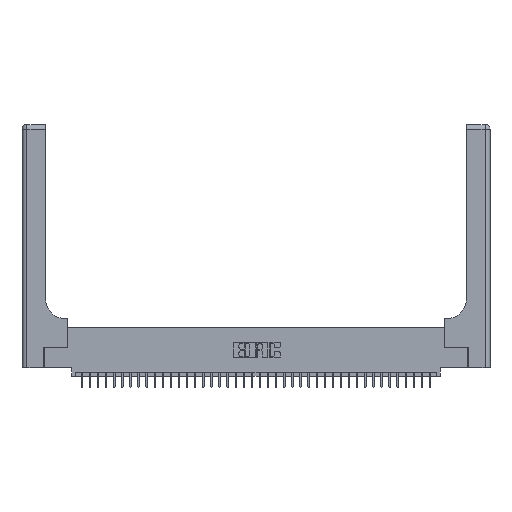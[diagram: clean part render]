
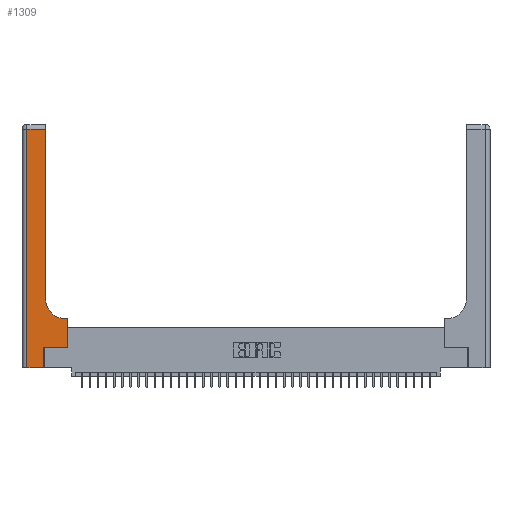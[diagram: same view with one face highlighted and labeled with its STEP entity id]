
A CAD part, top view. The second image highlights one B-rep face of the part: STEP entity #1309.
In plain terms, the highlighted planar face has unit normal (0, 0, 1).
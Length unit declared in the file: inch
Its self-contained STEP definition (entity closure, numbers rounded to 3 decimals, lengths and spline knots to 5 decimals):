
#410 = AXIS2_PLACEMENT_3D ( 'NONE', #12592, #3534, #15387 ) ;
#766 = DIRECTION ( 'NONE',  ( 0., 1., 0. ) ) ;
#1309 = ADVANCED_FACE ( 'NONE', ( #9378 ), #18802, .F. ) ;
#1773 = CARTESIAN_POINT ( 'NONE',  ( 0.06, 2.94, 0.37 ) ) ;
#2101 = LINE ( 'NONE', #14575, #7569 ) ;
#2392 = ORIENTED_EDGE ( 'NONE', *, *, #37537, .T. ) ;
#2927 = DIRECTION ( 'NONE',  ( 1., 0., 0. ) ) ;
#3534 = DIRECTION ( 'NONE',  ( 0., 0., -1. ) ) ;
#4312 = DIRECTION ( 'NONE',  ( 0., 1., 0. ) ) ;
#6578 = VECTOR ( 'NONE', #30595, 39.37008 ) ;
#6796 = VECTOR ( 'NONE', #11767, 39.37008 ) ;
#6918 = VECTOR ( 'NONE', #766, 39.37008 ) ;
#7103 = ORIENTED_EDGE ( 'NONE', *, *, #23775, .T. ) ;
#7121 = EDGE_CURVE ( 'NONE', #36727, #18903, #17304, .T. ) ;
#7472 = DIRECTION ( 'NONE',  ( -1., 0., 0. ) ) ;
#7569 = VECTOR ( 'NONE', #39627, 39.37008 ) ;
#7964 = VERTEX_POINT ( 'NONE', #16052 ) ;
#8925 = CARTESIAN_POINT ( 'NONE',  ( 0., 2.94, 0.37 ) ) ;
#9378 = FACE_OUTER_BOUND ( 'NONE', #26007, .T. ) ;
#11767 = DIRECTION ( 'NONE',  ( 1., 0., 0. ) ) ;
#12124 = VERTEX_POINT ( 'NONE', #19991 ) ;
#12384 = EDGE_CURVE ( 'NONE', #23441, #36727, #34752, .T. ) ;
#12592 = CARTESIAN_POINT ( 'NONE',  ( 0., 3., 0.37 ) ) ;
#13578 = EDGE_CURVE ( 'NONE', #18903, #12124, #34421, .T. ) ;
#14358 = ORIENTED_EDGE ( 'NONE', *, *, #38254, .T. ) ;
#14408 = LINE ( 'NONE', #20225, #29774 ) ;
#14575 = CARTESIAN_POINT ( 'NONE',  ( 0.269, 0.25, 0.37 ) ) ;
#14607 = ORIENTED_EDGE ( 'NONE', *, *, #31588, .T. ) ;
#14610 = ORIENTED_EDGE ( 'NONE', *, *, #13578, .T. ) ;
#15387 = DIRECTION ( 'NONE',  ( -1., 0., 0. ) ) ;
#16052 = CARTESIAN_POINT ( 'NONE',  ( 0.269, 0., 0.37 ) ) ;
#17304 = CIRCLE ( 'NONE', #26932, 0.25 ) ;
#18070 = EDGE_CURVE ( 'NONE', #12124, #37696, #33799, .T. ) ;
#18802 = PLANE ( 'NONE',  #410 ) ;
#18903 = VERTEX_POINT ( 'NONE', #23696 ) ;
#19710 = CARTESIAN_POINT ( 'NONE',  ( 0.2915, 0.6, 0.37 ) ) ;
#19991 = CARTESIAN_POINT ( 'NONE',  ( 0.2915, 2.94, 0.37 ) ) ;
#20225 = CARTESIAN_POINT ( 'NONE',  ( 0.5585, 0.25, 0.37 ) ) ;
#20835 = DIRECTION ( 'NONE',  ( 0., -1., 0. ) ) ;
#21014 = CARTESIAN_POINT ( 'NONE',  ( 0.5415, 0.85, 0.37 ) ) ;
#22218 = CARTESIAN_POINT ( 'NONE',  ( 0.06, 0., 0.37 ) ) ;
#22264 = LINE ( 'NONE', #37306, #6918 ) ;
#23161 = VECTOR ( 'NONE', #20835, 39.37008 ) ;
#23441 = VERTEX_POINT ( 'NONE', #26159 ) ;
#23696 = CARTESIAN_POINT ( 'NONE',  ( 0.2915, 0.85, 0.37 ) ) ;
#23775 = EDGE_CURVE ( 'NONE', #37696, #32423, #39291, .T. ) ;
#23808 = LINE ( 'NONE', #24216, #6796 ) ;
#24216 = CARTESIAN_POINT ( 'NONE',  ( 0., 0., 0.37 ) ) ;
#24341 = VERTEX_POINT ( 'NONE', #32307 ) ;
#25739 = CARTESIAN_POINT ( 'NONE',  ( 0.5585, 0.25, 0.37 ) ) ;
#26007 = EDGE_LOOP ( 'NONE', ( #14610, #33075, #7103, #27019, #2392, #14358, #14607, #39334, #32256 ) ) ;
#26159 = CARTESIAN_POINT ( 'NONE',  ( 0.5585, 0.6, 0.37 ) ) ;
#26932 = AXIS2_PLACEMENT_3D ( 'NONE', #21014, #33058, #2927 ) ;
#27019 = ORIENTED_EDGE ( 'NONE', *, *, #35331, .T. ) ;
#27295 = VECTOR ( 'NONE', #7472, 39.37008 ) ;
#27757 = VERTEX_POINT ( 'NONE', #25739 ) ;
#28258 = CARTESIAN_POINT ( 'NONE',  ( 0.5415, 0.6, 0.37 ) ) ;
#28415 = CARTESIAN_POINT ( 'NONE',  ( 0.2915, 3., 0.37 ) ) ;
#29774 = VECTOR ( 'NONE', #33050, 39.37008 ) ;
#29843 = VECTOR ( 'NONE', #4312, 39.37008 ) ;
#30595 = DIRECTION ( 'NONE',  ( -1., 0., 0. ) ) ;
#31588 = EDGE_CURVE ( 'NONE', #27757, #23441, #14408, .T. ) ;
#32256 = ORIENTED_EDGE ( 'NONE', *, *, #7121, .T. ) ;
#32307 = CARTESIAN_POINT ( 'NONE',  ( 0.269, 0.25, 0.37 ) ) ;
#32423 = VERTEX_POINT ( 'NONE', #22218 ) ;
#33050 = DIRECTION ( 'NONE',  ( 0., 1., 0. ) ) ;
#33058 = DIRECTION ( 'NONE',  ( 0., 0., -1. ) ) ;
#33075 = ORIENTED_EDGE ( 'NONE', *, *, #18070, .T. ) ;
#33083 = CARTESIAN_POINT ( 'NONE',  ( 0.06, 3., 0.37 ) ) ;
#33799 = LINE ( 'NONE', #8925, #6578 ) ;
#34421 = LINE ( 'NONE', #28415, #29843 ) ;
#34752 = LINE ( 'NONE', #19710, #27295 ) ;
#35331 = EDGE_CURVE ( 'NONE', #32423, #7964, #23808, .T. ) ;
#36727 = VERTEX_POINT ( 'NONE', #28258 ) ;
#37306 = CARTESIAN_POINT ( 'NONE',  ( 0.269, 0., 0.37 ) ) ;
#37537 = EDGE_CURVE ( 'NONE', #7964, #24341, #22264, .T. ) ;
#37696 = VERTEX_POINT ( 'NONE', #1773 ) ;
#38254 = EDGE_CURVE ( 'NONE', #24341, #27757, #2101, .T. ) ;
#39291 = LINE ( 'NONE', #33083, #23161 ) ;
#39334 = ORIENTED_EDGE ( 'NONE', *, *, #12384, .T. ) ;
#39627 = DIRECTION ( 'NONE',  ( 1., 0., 0. ) ) ;
